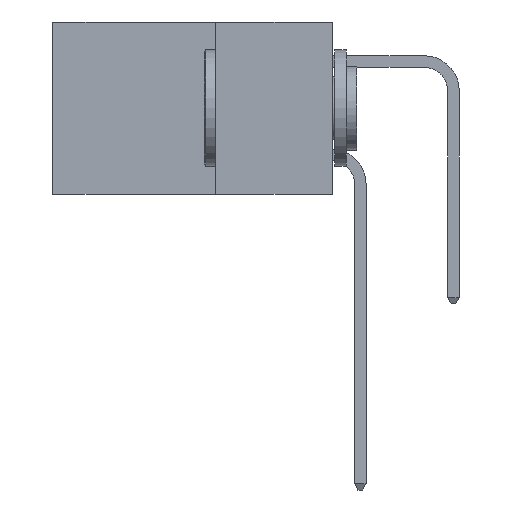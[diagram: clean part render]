
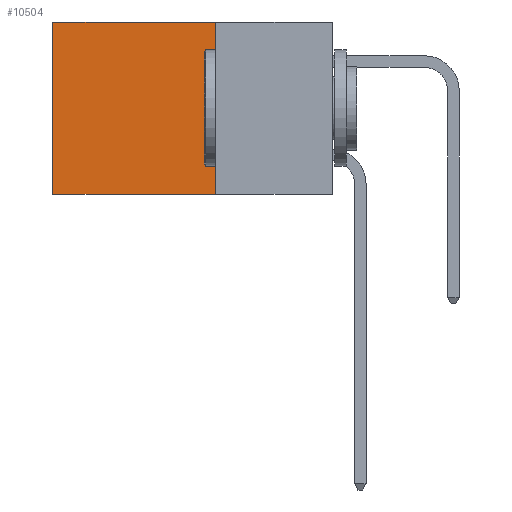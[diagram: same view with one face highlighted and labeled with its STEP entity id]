
A CAD part, left-side view. The second image highlights one B-rep face of the part: STEP entity #10504.
In plain terms, the highlighted planar face has unit normal (-1, 0, 0).
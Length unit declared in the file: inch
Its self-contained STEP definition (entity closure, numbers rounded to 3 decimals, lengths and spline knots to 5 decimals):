
#101 = CARTESIAN_POINT ( 'NONE',  ( 0.2615, 0.25, -0.37 ) ) ;
#128 = LINE ( 'NONE', #101, #12134 ) ;
#233 = CARTESIAN_POINT ( 'NONE',  ( 0.2615, 0.25, 0. ) ) ;
#1091 = VERTEX_POINT ( 'NONE', #1278 ) ;
#1278 = CARTESIAN_POINT ( 'NONE',  ( 0.2615, 0.6, -0.37 ) ) ;
#1762 = FACE_OUTER_BOUND ( 'NONE', #16017, .T. ) ;
#1864 = DIRECTION ( 'NONE',  ( 0., 0., -1. ) ) ;
#4654 = CARTESIAN_POINT ( 'NONE',  ( 0.2615, 0.25, -0.37 ) ) ;
#5130 = EDGE_CURVE ( 'NONE', #9603, #5806, #10777, .T. ) ;
#5781 = DIRECTION ( 'NONE',  ( 0., 1., 0. ) ) ;
#5804 = CARTESIAN_POINT ( 'NONE',  ( 0.2615, 0.25, -0.37 ) ) ;
#5806 = VERTEX_POINT ( 'NONE', #14756 ) ;
#6786 = VECTOR ( 'NONE', #20541, 39.37008 ) ;
#6806 = EDGE_CURVE ( 'NONE', #20178, #1091, #20489, .T. ) ;
#7283 = LINE ( 'NONE', #7996, #6786 ) ;
#7455 = ORIENTED_EDGE ( 'NONE', *, *, #14029, .T. ) ;
#7569 = ORIENTED_EDGE ( 'NONE', *, *, #5130, .T. ) ;
#7769 = AXIS2_PLACEMENT_3D ( 'NONE', #20588, #20490, #20487 ) ;
#7996 = CARTESIAN_POINT ( 'NONE',  ( 0.2615, 0.6, -0.37 ) ) ;
#9603 = VERTEX_POINT ( 'NONE', #20043 ) ;
#9618 = ORIENTED_EDGE ( 'NONE', *, *, #6806, .F. ) ;
#10504 = ADVANCED_FACE ( 'NONE', ( #1762 ), #20605, .F. ) ;
#10777 = LINE ( 'NONE', #233, #14489 ) ;
#10780 = ORIENTED_EDGE ( 'NONE', *, *, #18397, .F. ) ;
#12134 = VECTOR ( 'NONE', #1864, 39.37008 ) ;
#12194 = VECTOR ( 'NONE', #5781, 39.37008 ) ;
#14029 = EDGE_CURVE ( 'NONE', #5806, #1091, #7283, .T. ) ;
#14489 = VECTOR ( 'NONE', #17588, 39.37008 ) ;
#14756 = CARTESIAN_POINT ( 'NONE',  ( 0.2615, 0.6, 0. ) ) ;
#16017 = EDGE_LOOP ( 'NONE', ( #7455, #9618, #10780, #7569 ) ) ;
#17588 = DIRECTION ( 'NONE',  ( 0., 1., 0. ) ) ;
#18397 = EDGE_CURVE ( 'NONE', #9603, #20178, #128, .T. ) ;
#20043 = CARTESIAN_POINT ( 'NONE',  ( 0.2615, 0.25, 0. ) ) ;
#20178 = VERTEX_POINT ( 'NONE', #4654 ) ;
#20487 = DIRECTION ( 'NONE',  ( 0., 0., -1. ) ) ;
#20489 = LINE ( 'NONE', #5804, #12194 ) ;
#20490 = DIRECTION ( 'NONE',  ( 1., 0., 0. ) ) ;
#20541 = DIRECTION ( 'NONE',  ( 0., 0., -1. ) ) ;
#20588 = CARTESIAN_POINT ( 'NONE',  ( 0.2615, 0.25, -0.37 ) ) ;
#20605 = PLANE ( 'NONE',  #7769 ) ;
